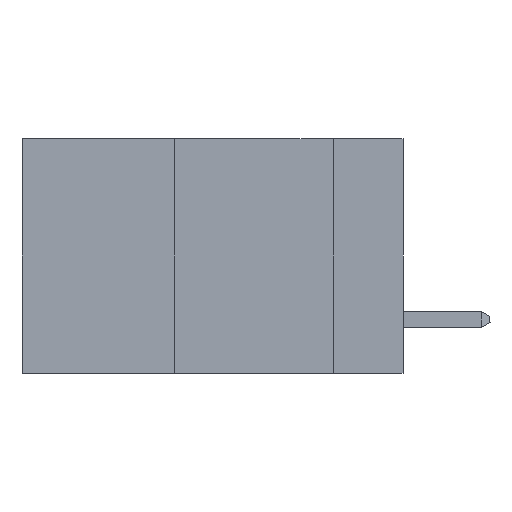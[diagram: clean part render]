
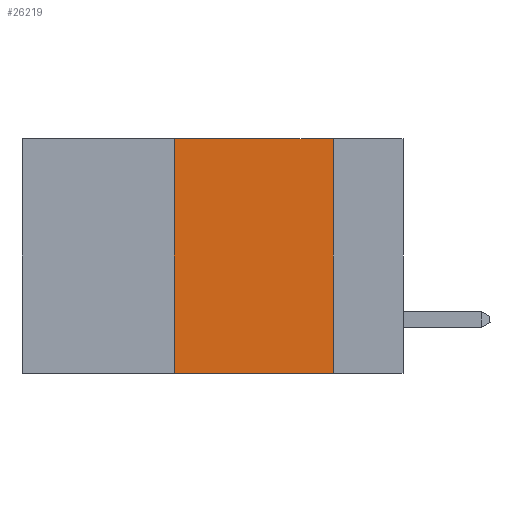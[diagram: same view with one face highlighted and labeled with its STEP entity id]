
A CAD part, left-side view. The second image highlights one B-rep face of the part: STEP entity #26219.
In plain terms, the highlighted planar face has unit normal (-1, 0, 0).
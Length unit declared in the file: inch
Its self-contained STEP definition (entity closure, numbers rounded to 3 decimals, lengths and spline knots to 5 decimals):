
#1110 = VECTOR ( 'NONE', #23478, 39.37008 ) ;
#1481 = VERTEX_POINT ( 'NONE', #8740 ) ;
#2680 = CARTESIAN_POINT ( 'NONE',  ( 0., 0.6, 0. ) ) ;
#4215 = FACE_OUTER_BOUND ( 'NONE', #37303, .T. ) ;
#6131 = VERTEX_POINT ( 'NONE', #26565 ) ;
#6267 = VECTOR ( 'NONE', #27428, 39.37008 ) ;
#8740 = CARTESIAN_POINT ( 'NONE',  ( 0., 0.11, -0.37 ) ) ;
#8830 = VERTEX_POINT ( 'NONE', #35417 ) ;
#9628 = CARTESIAN_POINT ( 'NONE',  ( 0., 0.36, 0. ) ) ;
#13790 = LINE ( 'NONE', #9628, #14328 ) ;
#14328 = VECTOR ( 'NONE', #34610, 39.37008 ) ;
#15638 = LINE ( 'NONE', #2680, #6267 ) ;
#17680 = VECTOR ( 'NONE', #20823, 39.37008 ) ;
#18677 = DIRECTION ( 'NONE',  ( 1., 0., 0. ) ) ;
#19424 = CARTESIAN_POINT ( 'NONE',  ( 0., 0.6, -0.37 ) ) ;
#19473 = ORIENTED_EDGE ( 'NONE', *, *, #42724, .F. ) ;
#20087 = EDGE_CURVE ( 'NONE', #38290, #1481, #38870, .T. ) ;
#20823 = DIRECTION ( 'NONE',  ( 0., 0., -1. ) ) ;
#21111 = ORIENTED_EDGE ( 'NONE', *, *, #44658, .F. ) ;
#22260 = CARTESIAN_POINT ( 'NONE',  ( 0., 0.6, 0. ) ) ;
#22376 = AXIS2_PLACEMENT_3D ( 'NONE', #22260, #18677, #32502 ) ;
#23478 = DIRECTION ( 'NONE',  ( 0., -1., 0. ) ) ;
#23964 = CARTESIAN_POINT ( 'NONE',  ( 0., 0.36, -0.37 ) ) ;
#26219 = ADVANCED_FACE ( 'NONE', ( #4215 ), #43397, .F. ) ;
#26565 = CARTESIAN_POINT ( 'NONE',  ( 0., 0.11, 0. ) ) ;
#27070 = LINE ( 'NONE', #31653, #17680 ) ;
#27428 = DIRECTION ( 'NONE',  ( 0., -1., 0. ) ) ;
#28815 = ORIENTED_EDGE ( 'NONE', *, *, #20087, .T. ) ;
#29699 = EDGE_CURVE ( 'NONE', #6131, #1481, #27070, .T. ) ;
#31653 = CARTESIAN_POINT ( 'NONE',  ( 0., 0.11, 0. ) ) ;
#32502 = DIRECTION ( 'NONE',  ( 0., 0., -1. ) ) ;
#32714 = ORIENTED_EDGE ( 'NONE', *, *, #29699, .F. ) ;
#34610 = DIRECTION ( 'NONE',  ( 0., 0., 1. ) ) ;
#35417 = CARTESIAN_POINT ( 'NONE',  ( 0., 0.36, 0. ) ) ;
#37303 = EDGE_LOOP ( 'NONE', ( #32714, #19473, #21111, #28815 ) ) ;
#38290 = VERTEX_POINT ( 'NONE', #23964 ) ;
#38870 = LINE ( 'NONE', #19424, #1110 ) ;
#42724 = EDGE_CURVE ( 'NONE', #8830, #6131, #15638, .T. ) ;
#43397 = PLANE ( 'NONE',  #22376 ) ;
#44658 = EDGE_CURVE ( 'NONE', #38290, #8830, #13790, .T. ) ;
